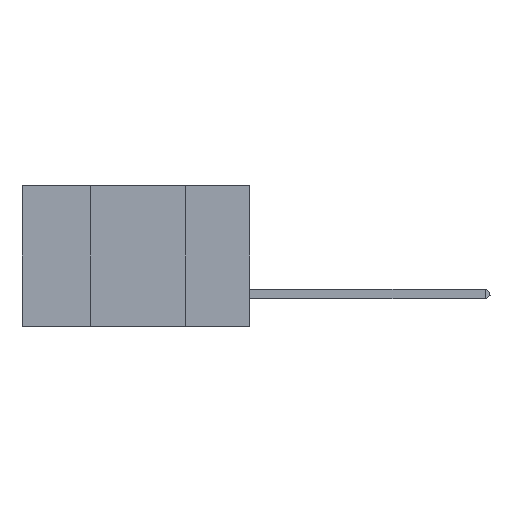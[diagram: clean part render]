
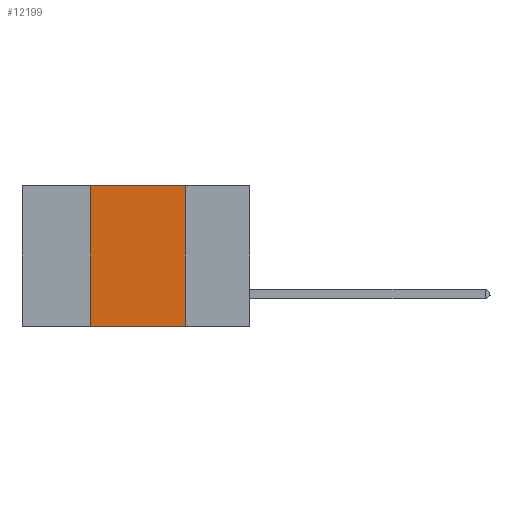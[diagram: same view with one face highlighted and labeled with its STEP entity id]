
A CAD part, left-side view. The second image highlights one B-rep face of the part: STEP entity #12199.
In plain terms, the highlighted planar face has unit normal (-1, 0, 0).
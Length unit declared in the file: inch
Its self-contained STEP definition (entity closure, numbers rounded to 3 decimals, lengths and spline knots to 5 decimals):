
#610 = AXIS2_PLACEMENT_3D ( 'NONE', #19354, #21195, #1079 ) ;
#1079 = DIRECTION ( 'NONE',  ( 0., 0., -1. ) ) ;
#2852 = CARTESIAN_POINT ( 'NONE',  ( 0., 0.17, -0.37 ) ) ;
#3279 = VERTEX_POINT ( 'NONE', #11799 ) ;
#3705 = EDGE_LOOP ( 'NONE', ( #6504, #11749, #18477, #7268 ) ) ;
#4068 = DIRECTION ( 'NONE',  ( 0., 0., -1. ) ) ;
#5575 = CARTESIAN_POINT ( 'NONE',  ( 0., 0.42, 0. ) ) ;
#5890 = VECTOR ( 'NONE', #13597, 39.37008 ) ;
#6460 = CARTESIAN_POINT ( 'NONE',  ( 0., 0.42, -0.37 ) ) ;
#6474 = EDGE_CURVE ( 'NONE', #14750, #25510, #18394, .T. ) ;
#6504 = ORIENTED_EDGE ( 'NONE', *, *, #6474, .F. ) ;
#7162 = VERTEX_POINT ( 'NONE', #6460 ) ;
#7268 = ORIENTED_EDGE ( 'NONE', *, *, #23416, .T. ) ;
#7491 = DIRECTION ( 'NONE',  ( 0., -1., 0. ) ) ;
#7540 = LINE ( 'NONE', #5575, #5890 ) ;
#8598 = VECTOR ( 'NONE', #4068, 39.37008 ) ;
#9668 = VECTOR ( 'NONE', #12936, 39.37008 ) ;
#10075 = VECTOR ( 'NONE', #7491, 39.37008 ) ;
#11222 = LINE ( 'NONE', #25163, #9668 ) ;
#11749 = ORIENTED_EDGE ( 'NONE', *, *, #24141, .F. ) ;
#11799 = CARTESIAN_POINT ( 'NONE',  ( 0., 0.42, 0. ) ) ;
#12199 = ADVANCED_FACE ( 'NONE', ( #23032 ), #15153, .F. ) ;
#12936 = DIRECTION ( 'NONE',  ( 0., -1., 0. ) ) ;
#13597 = DIRECTION ( 'NONE',  ( 0., 0., 1. ) ) ;
#13806 = CARTESIAN_POINT ( 'NONE',  ( 0., 0.17, 0. ) ) ;
#14750 = VERTEX_POINT ( 'NONE', #13806 ) ;
#15153 = PLANE ( 'NONE',  #610 ) ;
#17374 = EDGE_CURVE ( 'NONE', #7162, #3279, #7540, .T. ) ;
#18394 = LINE ( 'NONE', #22192, #8598 ) ;
#18477 = ORIENTED_EDGE ( 'NONE', *, *, #17374, .F. ) ;
#19354 = CARTESIAN_POINT ( 'NONE',  ( 0., 0.6, 0. ) ) ;
#19988 = CARTESIAN_POINT ( 'NONE',  ( 0., 0.6, -0.37 ) ) ;
#21195 = DIRECTION ( 'NONE',  ( 1., 0., 0. ) ) ;
#21702 = LINE ( 'NONE', #19988, #10075 ) ;
#22192 = CARTESIAN_POINT ( 'NONE',  ( 0., 0.17, 0. ) ) ;
#23032 = FACE_OUTER_BOUND ( 'NONE', #3705, .T. ) ;
#23416 = EDGE_CURVE ( 'NONE', #7162, #25510, #21702, .T. ) ;
#24141 = EDGE_CURVE ( 'NONE', #3279, #14750, #11222, .T. ) ;
#25163 = CARTESIAN_POINT ( 'NONE',  ( 0., 0.6, 0. ) ) ;
#25510 = VERTEX_POINT ( 'NONE', #2852 ) ;
